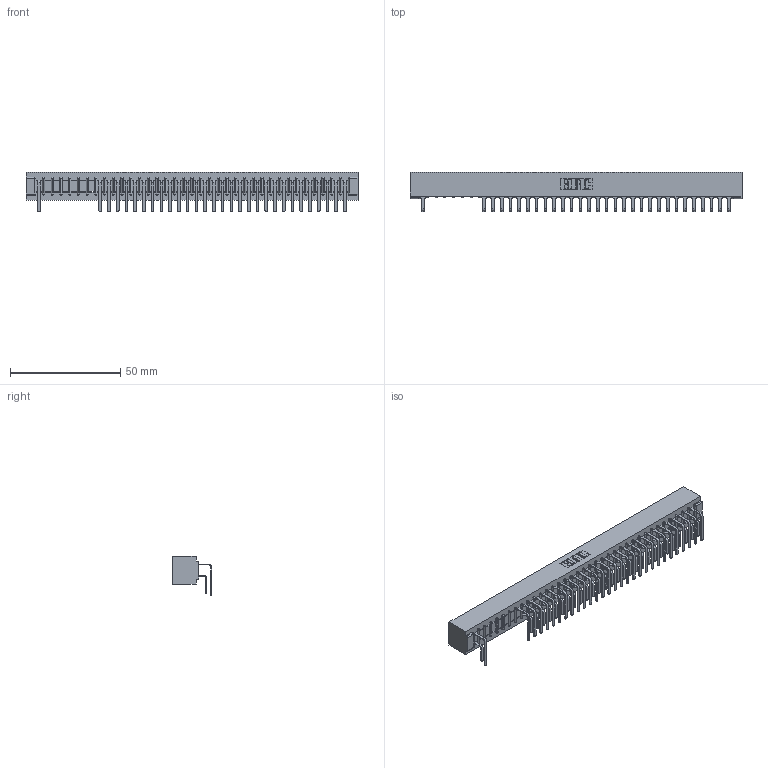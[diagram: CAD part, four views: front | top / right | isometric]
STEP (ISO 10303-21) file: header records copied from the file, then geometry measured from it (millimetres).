
FILE_DESCRIPTION (( 'STEP AP203' ), '1' );
FILE_NAME ('307-036-559-101.STEP', '2018-08-05T08:14:26', ( '' ), ( '' ), 'SwSTEP 2.0', 'SolidWorks 2016', '' );
FILE_SCHEMA (( 'CONFIG_CONTROL_DESIGN' ));
Length unit declared in the file: inch
Products named in the file (4): 307 Part_No Mounting Lugs; 307-290-001_558 559 - 1 (Single); 307-290-001_559 - 2 (Single); 307-036-559-101
Assembly tree (60 placements, depth 2):
  307-036-559-101
    307 Part_No Mounting Lugs
    307-290-001_558 559 - 1 (Single)  x29
    307-290-001_559 - 2 (Single)  x30
Bounding box: 150.52 x 17.69 x 18.07 mm (x, y, z)
Volume: 16606 mm3; surface area: 20941.5 mm2
Topology: 60 solids, 60 shells, 3227 faces, 9093 edges, 5882 vertices
Faces by surface type: plane 2091, cylinder 1062, sphere 74
Entity records: 33507 total; most frequent: CARTESIAN_POINT 5537, ORIENTED_EDGE 5498, DIRECTION 5411, EDGE_CURVE 2749, VECTOR 2107, LINE 2107, VERTEX_POINT 1778, AXIS2_PLACEMENT_3D 1652
